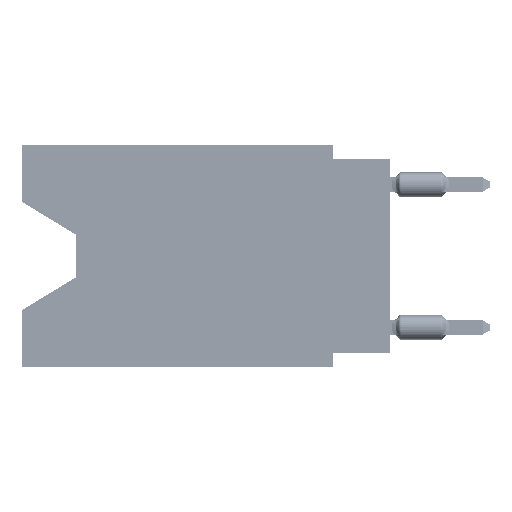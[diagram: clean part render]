
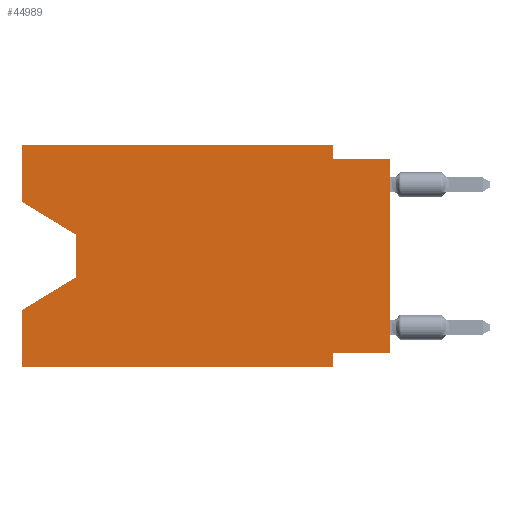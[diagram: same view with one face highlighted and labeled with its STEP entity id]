
A CAD part, left-side view. The second image highlights one B-rep face of the part: STEP entity #44989.
In plain terms, the highlighted planar face has unit normal (-1, 0, 0).
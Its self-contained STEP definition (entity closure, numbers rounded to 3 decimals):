
#231 = ORIENTED_EDGE ( 'NONE', *, *, #73699, .F. ) ;
#763 = ORIENTED_EDGE ( 'NONE', *, *, #18630, .T. ) ;
#1530 = VERTEX_POINT ( 'NONE', #21324 ) ;
#2694 = DIRECTION ( 'NONE',  ( 1., 0., 0. ) ) ;
#3515 = VERTEX_POINT ( 'NONE', #8964 ) ;
#4511 = LINE ( 'NONE', #4912, #40098 ) ;
#4546 = VECTOR ( 'NONE', #16373, 1000. ) ;
#4647 = DIRECTION ( 'NONE',  ( 0., -0.855, -0.519 ) ) ;
#4912 = CARTESIAN_POINT ( 'NONE',  ( 0., 2.54, 0. ) ) ;
#5265 = VERTEX_POINT ( 'NONE', #9463 ) ;
#8263 = EDGE_CURVE ( 'NONE', #50984, #3515, #73127, .T. ) ;
#8964 = CARTESIAN_POINT ( 'NONE',  ( 0., 0., -0.635 ) ) ;
#9318 = PLANE ( 'NONE',  #28685 ) ;
#9463 = CARTESIAN_POINT ( 'NONE',  ( 0., 0., -9.271 ) ) ;
#11464 = CARTESIAN_POINT ( 'NONE',  ( 0., 16.383, -7.36 ) ) ;
#12671 = LINE ( 'NONE', #66364, #42286 ) ;
#15187 = CARTESIAN_POINT ( 'NONE',  ( 0., 2.54, -9.906 ) ) ;
#15723 = VERTEX_POINT ( 'NONE', #19680 ) ;
#16373 = DIRECTION ( 'NONE',  ( 0., 1., 0. ) ) ;
#17315 = CARTESIAN_POINT ( 'NONE',  ( 0., 16.383, 0. ) ) ;
#18630 = EDGE_CURVE ( 'NONE', #50889, #37937, #12671, .T. ) ;
#18785 = CARTESIAN_POINT ( 'NONE',  ( 0., 13.97, -4.013 ) ) ;
#19449 = DIRECTION ( 'NONE',  ( 0., -1., 0. ) ) ;
#19680 = CARTESIAN_POINT ( 'NONE',  ( 0., 2.54, 0. ) ) ;
#20884 = ORIENTED_EDGE ( 'NONE', *, *, #55139, .T. ) ;
#20892 = VECTOR ( 'NONE', #69247, 1000. ) ;
#20912 = LINE ( 'NONE', #57724, #66036 ) ;
#21324 = CARTESIAN_POINT ( 'NONE',  ( 0., 13.97, -5.893 ) ) ;
#22253 = CARTESIAN_POINT ( 'NONE',  ( 0., 16.383, -2.546 ) ) ;
#22615 = VERTEX_POINT ( 'NONE', #75078 ) ;
#23598 = CARTESIAN_POINT ( 'NONE',  ( 0., 13.97, -4.013 ) ) ;
#24957 = ORIENTED_EDGE ( 'NONE', *, *, #53733, .F. ) ;
#24976 = EDGE_CURVE ( 'NONE', #71579, #29709, #44240, .T. ) ;
#25137 = LINE ( 'NONE', #43141, #70071 ) ;
#25586 = DIRECTION ( 'NONE',  ( 0., -1., 0. ) ) ;
#26391 = EDGE_CURVE ( 'NONE', #15723, #50984, #4511, .T. ) ;
#26940 = CARTESIAN_POINT ( 'NONE',  ( 0., 16.383, -2.546 ) ) ;
#27334 = ORIENTED_EDGE ( 'NONE', *, *, #39561, .F. ) ;
#28403 = CARTESIAN_POINT ( 'NONE',  ( 0., 16.383, -9.906 ) ) ;
#28685 = AXIS2_PLACEMENT_3D ( 'NONE', #61458, #2694, #57133 ) ;
#29369 = VECTOR ( 'NONE', #39004, 1000. ) ;
#29709 = VERTEX_POINT ( 'NONE', #50919 ) ;
#32410 = ORIENTED_EDGE ( 'NONE', *, *, #76504, .T. ) ;
#33051 = VECTOR ( 'NONE', #19449, 1000. ) ;
#35172 = EDGE_CURVE ( 'NONE', #1530, #49861, #20912, .T. ) ;
#37915 = EDGE_CURVE ( 'NONE', #62297, #1530, #67341, .T. ) ;
#37937 = VERTEX_POINT ( 'NONE', #43029 ) ;
#38426 = DIRECTION ( 'NONE',  ( 0., 0., 1. ) ) ;
#38767 = DIRECTION ( 'NONE',  ( 0., 0., 1. ) ) ;
#39004 = DIRECTION ( 'NONE',  ( 0., 0., -1. ) ) ;
#39561 = EDGE_CURVE ( 'NONE', #5265, #22615, #57918, .T. ) ;
#39956 = LINE ( 'NONE', #51730, #76218 ) ;
#40098 = VECTOR ( 'NONE', #52680, 1000. ) ;
#40642 = CARTESIAN_POINT ( 'NONE',  ( 0., 0., -9.271 ) ) ;
#40835 = ORIENTED_EDGE ( 'NONE', *, *, #72810, .F. ) ;
#40840 = VECTOR ( 'NONE', #53355, 1000. ) ;
#42286 = VECTOR ( 'NONE', #25586, 1000. ) ;
#43029 = CARTESIAN_POINT ( 'NONE',  ( 0., 2.54, -9.906 ) ) ;
#43141 = CARTESIAN_POINT ( 'NONE',  ( 0., 16.383, 0. ) ) ;
#44240 = LINE ( 'NONE', #62678, #63805 ) ;
#44989 = ADVANCED_FACE ( 'NONE', ( #69259 ), #9318, .F. ) ;
#46027 = ORIENTED_EDGE ( 'NONE', *, *, #35172, .T. ) ;
#46412 = CARTESIAN_POINT ( 'NONE',  ( 0., 2.54, -0.635 ) ) ;
#47881 = DIRECTION ( 'NONE',  ( 0., -1., 0. ) ) ;
#49861 = VERTEX_POINT ( 'NONE', #11464 ) ;
#50889 = VERTEX_POINT ( 'NONE', #28403 ) ;
#50919 = CARTESIAN_POINT ( 'NONE',  ( 0., 16.383, 0. ) ) ;
#50984 = VERTEX_POINT ( 'NONE', #46412 ) ;
#51730 = CARTESIAN_POINT ( 'NONE',  ( 0., 0., 0. ) ) ;
#52663 = EDGE_LOOP ( 'NONE', ( #20884, #57972, #46027, #231, #763, #40835, #27334, #32410, #67670, #61911, #24957, #70685 ) ) ;
#52680 = DIRECTION ( 'NONE',  ( 0., 0., -1. ) ) ;
#53355 = DIRECTION ( 'NONE',  ( 0., 0., 1. ) ) ;
#53733 = EDGE_CURVE ( 'NONE', #29709, #15723, #25137, .T. ) ;
#54745 = CARTESIAN_POINT ( 'NONE',  ( 0., 0., -0.635 ) ) ;
#55139 = EDGE_CURVE ( 'NONE', #71579, #62297, #58302, .T. ) ;
#56462 = VECTOR ( 'NONE', #4647, 1000. ) ;
#57133 = DIRECTION ( 'NONE',  ( 0., 0., -1. ) ) ;
#57724 = CARTESIAN_POINT ( 'NONE',  ( 0., 13.97, -5.893 ) ) ;
#57918 = LINE ( 'NONE', #40642, #4546 ) ;
#57972 = ORIENTED_EDGE ( 'NONE', *, *, #37915, .T. ) ;
#58302 = LINE ( 'NONE', #22253, #56462 ) ;
#61458 = CARTESIAN_POINT ( 'NONE',  ( 0., 16.383, 0. ) ) ;
#61911 = ORIENTED_EDGE ( 'NONE', *, *, #26391, .F. ) ;
#62297 = VERTEX_POINT ( 'NONE', #23598 ) ;
#62678 = CARTESIAN_POINT ( 'NONE',  ( 0., 16.383, 0. ) ) ;
#63614 = DIRECTION ( 'NONE',  ( 0., 0.855, -0.519 ) ) ;
#63805 = VECTOR ( 'NONE', #38767, 1000. ) ;
#64737 = LINE ( 'NONE', #17315, #40840 ) ;
#66036 = VECTOR ( 'NONE', #63614, 1000. ) ;
#66364 = CARTESIAN_POINT ( 'NONE',  ( 0., 16.383, -9.906 ) ) ;
#67341 = LINE ( 'NONE', #18785, #29369 ) ;
#67670 = ORIENTED_EDGE ( 'NONE', *, *, #8263, .F. ) ;
#68876 = LINE ( 'NONE', #15187, #20892 ) ;
#69247 = DIRECTION ( 'NONE',  ( 0., 0., -1. ) ) ;
#69259 = FACE_OUTER_BOUND ( 'NONE', #52663, .T. ) ;
#70071 = VECTOR ( 'NONE', #47881, 1000. ) ;
#70685 = ORIENTED_EDGE ( 'NONE', *, *, #24976, .F. ) ;
#71579 = VERTEX_POINT ( 'NONE', #26940 ) ;
#72810 = EDGE_CURVE ( 'NONE', #22615, #37937, #68876, .T. ) ;
#73127 = LINE ( 'NONE', #54745, #33051 ) ;
#73699 = EDGE_CURVE ( 'NONE', #50889, #49861, #64737, .T. ) ;
#75078 = CARTESIAN_POINT ( 'NONE',  ( 0., 2.54, -9.271 ) ) ;
#76218 = VECTOR ( 'NONE', #38426, 1000. ) ;
#76504 = EDGE_CURVE ( 'NONE', #5265, #3515, #39956, .T. ) ;
